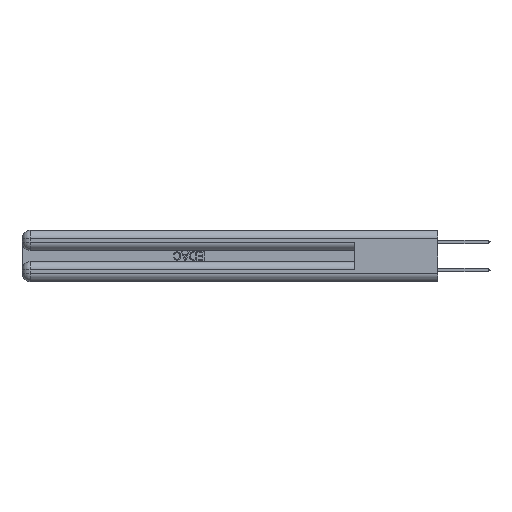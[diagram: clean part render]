
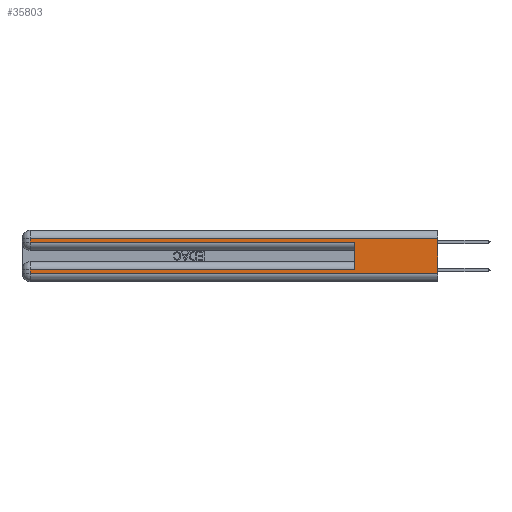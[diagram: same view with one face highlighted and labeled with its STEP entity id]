
A CAD part, left-side view. The second image highlights one B-rep face of the part: STEP entity #35803.
In plain terms, the highlighted planar face has unit normal (-1, 0, 0).
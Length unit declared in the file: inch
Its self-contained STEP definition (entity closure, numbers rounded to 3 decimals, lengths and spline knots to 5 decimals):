
#251 = PLANE ( 'NONE',  #44426 ) ;
#935 = VERTEX_POINT ( 'NONE', #15035 ) ;
#2093 = VERTEX_POINT ( 'NONE', #32669 ) ;
#3331 = DIRECTION ( 'NONE',  ( 0., 1., 0. ) ) ;
#4021 = DIRECTION ( 'NONE',  ( 0., 0., -1. ) ) ;
#4985 = VECTOR ( 'NONE', #24928, 39.37008 ) ;
#5321 = DIRECTION ( 'NONE',  ( 0., 0., -1. ) ) ;
#5702 = ORIENTED_EDGE ( 'NONE', *, *, #25335, .T. ) ;
#6048 = ORIENTED_EDGE ( 'NONE', *, *, #21425, .F. ) ;
#6050 = CARTESIAN_POINT ( 'NONE',  ( 0., 2.94, 0.37 ) ) ;
#6458 = ORIENTED_EDGE ( 'NONE', *, *, #18214, .T. ) ;
#6479 = VECTOR ( 'NONE', #13934, 39.37008 ) ;
#6594 = CARTESIAN_POINT ( 'NONE',  ( 0., 0.6, 0.085 ) ) ;
#6666 = EDGE_CURVE ( 'NONE', #9137, #2093, #31531, .T. ) ;
#6831 = ORIENTED_EDGE ( 'NONE', *, *, #6666, .T. ) ;
#7586 = EDGE_CURVE ( 'NONE', #45277, #9137, #32588, .T. ) ;
#8723 = CARTESIAN_POINT ( 'NONE',  ( 0., 0., 0.06 ) ) ;
#9137 = VERTEX_POINT ( 'NONE', #45322 ) ;
#9332 = EDGE_CURVE ( 'NONE', #37640, #45277, #32418, .T. ) ;
#9542 = ORIENTED_EDGE ( 'NONE', *, *, #9906, .T. ) ;
#9906 = EDGE_CURVE ( 'NONE', #935, #39301, #28832, .T. ) ;
#10162 = VECTOR ( 'NONE', #14333, 39.37008 ) ;
#10690 = CARTESIAN_POINT ( 'NONE',  ( 0., 0., 0.06 ) ) ;
#11462 = VECTOR ( 'NONE', #19295, 39.37008 ) ;
#13934 = DIRECTION ( 'NONE',  ( 0., 0., -1. ) ) ;
#14333 = DIRECTION ( 'NONE',  ( 0., 1., 0. ) ) ;
#14713 = VERTEX_POINT ( 'NONE', #8723 ) ;
#15035 = CARTESIAN_POINT ( 'NONE',  ( 0., 2.94, 0.085 ) ) ;
#18214 = EDGE_CURVE ( 'NONE', #39301, #14713, #32257, .T. ) ;
#18315 = CARTESIAN_POINT ( 'NONE',  ( 0., 0., 0.31 ) ) ;
#19186 = CARTESIAN_POINT ( 'NONE',  ( 0., 2.94, 0.31 ) ) ;
#19295 = DIRECTION ( 'NONE',  ( 0., -1., 0. ) ) ;
#21241 = FACE_OUTER_BOUND ( 'NONE', #38073, .T. ) ;
#21425 = EDGE_CURVE ( 'NONE', #31625, #2093, #34947, .T. ) ;
#22292 = VECTOR ( 'NONE', #29658, 39.37008 ) ;
#23617 = CARTESIAN_POINT ( 'NONE',  ( 0., 2.94, 0.06 ) ) ;
#24061 = CARTESIAN_POINT ( 'NONE',  ( 0., 0., 0.37 ) ) ;
#24928 = DIRECTION ( 'NONE',  ( 0., 0., 1. ) ) ;
#25335 = EDGE_CURVE ( 'NONE', #31625, #935, #47779, .T. ) ;
#26562 = DIRECTION ( 'NONE',  ( 1., 0., 0. ) ) ;
#28357 = ORIENTED_EDGE ( 'NONE', *, *, #34125, .F. ) ;
#28832 = LINE ( 'NONE', #43990, #6479 ) ;
#29629 = CARTESIAN_POINT ( 'NONE',  ( 0., 0., 0.31 ) ) ;
#29658 = DIRECTION ( 'NONE',  ( 0., -1., 0. ) ) ;
#30276 = VECTOR ( 'NONE', #32335, 39.37008 ) ;
#31531 = LINE ( 'NONE', #37978, #11462 ) ;
#31625 = VERTEX_POINT ( 'NONE', #6594 ) ;
#32257 = LINE ( 'NONE', #10690, #22292 ) ;
#32335 = DIRECTION ( 'NONE',  ( 0., 0., -1. ) ) ;
#32418 = LINE ( 'NONE', #29629, #41209 ) ;
#32588 = LINE ( 'NONE', #6050, #30276 ) ;
#32669 = CARTESIAN_POINT ( 'NONE',  ( 0., 0.6, 0.285 ) ) ;
#34125 = EDGE_CURVE ( 'NONE', #37640, #14713, #42429, .T. ) ;
#34947 = LINE ( 'NONE', #47362, #4985 ) ;
#35803 = ADVANCED_FACE ( 'NONE', ( #21241 ), #251, .F. ) ;
#37640 = VERTEX_POINT ( 'NONE', #18315 ) ;
#37662 = CARTESIAN_POINT ( 'NONE',  ( 0., 0., 0.37 ) ) ;
#37767 = ORIENTED_EDGE ( 'NONE', *, *, #7586, .T. ) ;
#37978 = CARTESIAN_POINT ( 'NONE',  ( 0., 0., 0.285 ) ) ;
#38073 = EDGE_LOOP ( 'NONE', ( #28357, #38392, #37767, #6831, #6048, #5702, #9542, #6458 ) ) ;
#38392 = ORIENTED_EDGE ( 'NONE', *, *, #9332, .T. ) ;
#39301 = VERTEX_POINT ( 'NONE', #23617 ) ;
#41209 = VECTOR ( 'NONE', #3331, 39.37008 ) ;
#41255 = VECTOR ( 'NONE', #5321, 39.37008 ) ;
#42429 = LINE ( 'NONE', #24061, #41255 ) ;
#43990 = CARTESIAN_POINT ( 'NONE',  ( 0., 2.94, 0.37 ) ) ;
#44386 = CARTESIAN_POINT ( 'NONE',  ( 0., 0., 0.085 ) ) ;
#44426 = AXIS2_PLACEMENT_3D ( 'NONE', #37662, #26562, #4021 ) ;
#45277 = VERTEX_POINT ( 'NONE', #19186 ) ;
#45322 = CARTESIAN_POINT ( 'NONE',  ( 0., 2.94, 0.285 ) ) ;
#47362 = CARTESIAN_POINT ( 'NONE',  ( 0., 0.6, 0.145 ) ) ;
#47779 = LINE ( 'NONE', #44386, #10162 ) ;
